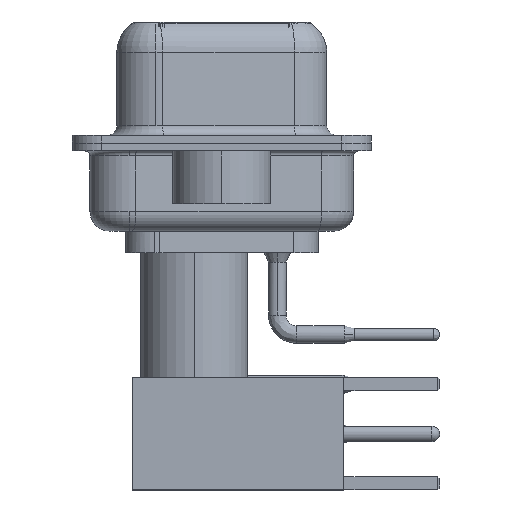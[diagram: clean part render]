
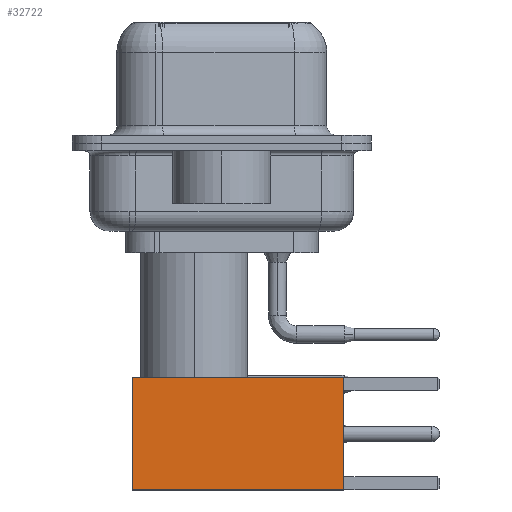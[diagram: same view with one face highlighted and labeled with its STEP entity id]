
A CAD part, left-side view. The second image highlights one B-rep face of the part: STEP entity #32722.
In plain terms, the highlighted face is planar.
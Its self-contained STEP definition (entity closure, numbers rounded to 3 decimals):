
#456 = EDGE_CURVE ( 'NONE', #4339, #2249, #16851, .T. ) ;
#790 = FACE_OUTER_BOUND ( 'NONE', #20964, .T. ) ;
#1297 = LINE ( 'NONE', #1660, #2909 ) ;
#1660 = CARTESIAN_POINT ( 'NONE',  ( 2.875, 2.875, 0. ) ) ;
#2249 = VERTEX_POINT ( 'NONE', #32806 ) ;
#2608 = VECTOR ( 'NONE', #8378, 1000. ) ;
#2809 = DIRECTION ( 'NONE',  ( 0., 1., 0. ) ) ;
#2909 = VECTOR ( 'NONE', #20787, 1000. ) ;
#2971 = CARTESIAN_POINT ( 'NONE',  ( 2.875, 2.875, 10.82 ) ) ;
#4339 = VERTEX_POINT ( 'NONE', #2971 ) ;
#8138 = ORIENTED_EDGE ( 'NONE', *, *, #31727, .T. ) ;
#8378 = DIRECTION ( 'NONE',  ( -1., 0., 0. ) ) ;
#8697 = DIRECTION ( 'NONE',  ( 0., 0., -1. ) ) ;
#8810 = AXIS2_PLACEMENT_3D ( 'NONE', #11932, #2809, #30803 ) ;
#11932 = CARTESIAN_POINT ( 'NONE',  ( 2.875, 2.875, 0. ) ) ;
#12088 = VECTOR ( 'NONE', #8697, 1000. ) ;
#14064 = EDGE_CURVE ( 'NONE', #2249, #21430, #14531, .T. ) ;
#14384 = CARTESIAN_POINT ( 'NONE',  ( 0., 2.875, 0. ) ) ;
#14531 = LINE ( 'NONE', #31033, #12088 ) ;
#16851 = LINE ( 'NONE', #19058, #23569 ) ;
#19058 = CARTESIAN_POINT ( 'NONE',  ( 0., 2.875, 10.82 ) ) ;
#20322 = CARTESIAN_POINT ( 'NONE',  ( -2.875, 2.875, 0. ) ) ;
#20787 = DIRECTION ( 'NONE',  ( 0., 0., -1. ) ) ;
#20964 = EDGE_LOOP ( 'NONE', ( #8138, #31365, #23762, #27794 ) ) ;
#21430 = VERTEX_POINT ( 'NONE', #20322 ) ;
#21811 = VERTEX_POINT ( 'NONE', #30263 ) ;
#22894 = EDGE_CURVE ( 'NONE', #21811, #21430, #26300, .T. ) ;
#23569 = VECTOR ( 'NONE', #30460, 1000. ) ;
#23762 = ORIENTED_EDGE ( 'NONE', *, *, #14064, .F. ) ;
#26300 = LINE ( 'NONE', #14384, #2608 ) ;
#27794 = ORIENTED_EDGE ( 'NONE', *, *, #456, .F. ) ;
#30263 = CARTESIAN_POINT ( 'NONE',  ( 2.875, 2.875, 0. ) ) ;
#30460 = DIRECTION ( 'NONE',  ( -1., 0., 0. ) ) ;
#30803 = DIRECTION ( 'NONE',  ( 0., 0., 1. ) ) ;
#31033 = CARTESIAN_POINT ( 'NONE',  ( -2.875, 2.875, 0. ) ) ;
#31365 = ORIENTED_EDGE ( 'NONE', *, *, #22894, .T. ) ;
#31727 = EDGE_CURVE ( 'NONE', #4339, #21811, #1297, .T. ) ;
#32722 = ADVANCED_FACE ( 'NONE', ( #790 ), #33541, .T. ) ;
#32806 = CARTESIAN_POINT ( 'NONE',  ( -2.875, 2.875, 10.82 ) ) ;
#33541 = PLANE ( 'NONE',  #8810 ) ;
